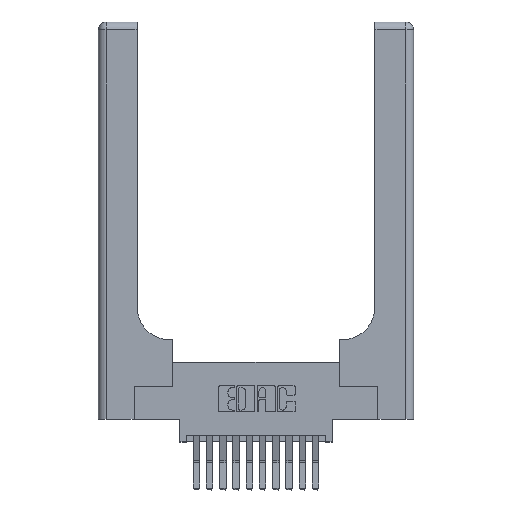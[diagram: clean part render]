
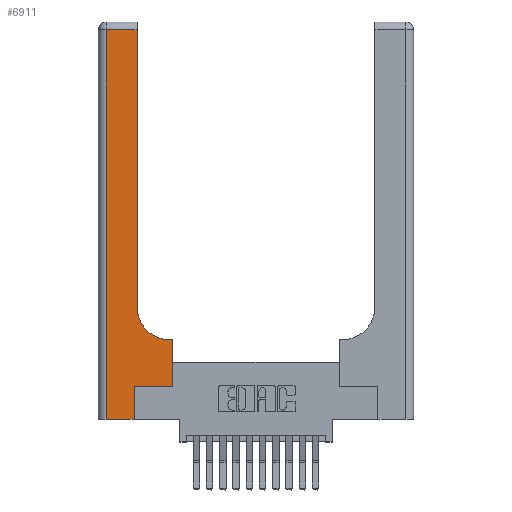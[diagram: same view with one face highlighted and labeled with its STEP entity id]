
A CAD part, top view. The second image highlights one B-rep face of the part: STEP entity #6911.
In plain terms, the highlighted planar face has unit normal (0, 0, 1).
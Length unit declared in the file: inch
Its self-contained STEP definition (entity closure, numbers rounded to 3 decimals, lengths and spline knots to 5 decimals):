
#152 = ORIENTED_EDGE ( 'NONE', *, *, #15202, .T. ) ;
#239 = ORIENTED_EDGE ( 'NONE', *, *, #14470, .T. ) ;
#265 = ORIENTED_EDGE ( 'NONE', *, *, #12878, .T. ) ;
#397 = ORIENTED_EDGE ( 'NONE', *, *, #15425, .T. ) ;
#580 = CARTESIAN_POINT ( 'NONE',  ( 0.269, 0., 0.37 ) ) ;
#607 = CARTESIAN_POINT ( 'NONE',  ( 0.2915, 3., 0.37 ) ) ;
#729 = ORIENTED_EDGE ( 'NONE', *, *, #12782, .T. ) ;
#766 = VECTOR ( 'NONE', #2302, 39.37008 ) ;
#855 = ORIENTED_EDGE ( 'NONE', *, *, #3325, .T. ) ;
#947 = ORIENTED_EDGE ( 'NONE', *, *, #1879, .T. ) ;
#1004 = ORIENTED_EDGE ( 'NONE', *, *, #9409, .T. ) ;
#1080 = ORIENTED_EDGE ( 'NONE', *, *, #13594, .T. ) ;
#1739 = CARTESIAN_POINT ( 'NONE',  ( 0.5585, 0.25, 0.37 ) ) ;
#1879 = EDGE_CURVE ( 'NONE', #11825, #15811, #7840, .T. ) ;
#2097 = VECTOR ( 'NONE', #4702, 39.37008 ) ;
#2302 = DIRECTION ( 'NONE',  ( 0., -1., 0. ) ) ;
#2559 = VECTOR ( 'NONE', #10254, 39.37008 ) ;
#2686 = VECTOR ( 'NONE', #6074, 39.37008 ) ;
#2848 = CARTESIAN_POINT ( 'NONE',  ( 0.06, 2.94, 0.37 ) ) ;
#3325 = EDGE_CURVE ( 'NONE', #12259, #11825, #9900, .T. ) ;
#3659 = CARTESIAN_POINT ( 'NONE',  ( 0.269, 0.25, 0.37 ) ) ;
#3710 = DIRECTION ( 'NONE',  ( 1., 0., 0. ) ) ;
#3801 = CARTESIAN_POINT ( 'NONE',  ( 0., 0., 0.37 ) ) ;
#3952 = CARTESIAN_POINT ( 'NONE',  ( 0.5415, 0.6, 0.37 ) ) ;
#4039 = DIRECTION ( 'NONE',  ( 0., 0., -1. ) ) ;
#4230 = VERTEX_POINT ( 'NONE', #2848 ) ;
#4231 = VERTEX_POINT ( 'NONE', #14883 ) ;
#4249 = VECTOR ( 'NONE', #15240, 39.37008 ) ;
#4646 = LINE ( 'NONE', #607, #15344 ) ;
#4690 = VERTEX_POINT ( 'NONE', #3952 ) ;
#4702 = DIRECTION ( 'NONE',  ( -1., 0., 0. ) ) ;
#4704 = CARTESIAN_POINT ( 'NONE',  ( 0.2915, 0.6, 0.37 ) ) ;
#5261 = LINE ( 'NONE', #3801, #8450 ) ;
#5728 = LINE ( 'NONE', #8730, #2097 ) ;
#6055 = EDGE_LOOP ( 'NONE', ( #152, #239, #265, #397, #729, #855, #947, #1004, #1080 ) ) ;
#6074 = DIRECTION ( 'NONE',  ( -1., 0., 0. ) ) ;
#6312 = VECTOR ( 'NONE', #3710, 39.37008 ) ;
#6911 = ADVANCED_FACE ( 'NONE', ( #14519 ), #11009, .F. ) ;
#7008 = DIRECTION ( 'NONE',  ( 0., 0., -1. ) ) ;
#7840 = LINE ( 'NONE', #1739, #4249 ) ;
#7886 = AXIS2_PLACEMENT_3D ( 'NONE', #12119, #4039, #13439 ) ;
#8450 = VECTOR ( 'NONE', #15857, 39.37008 ) ;
#8522 = CIRCLE ( 'NONE', #7886, 0.25 ) ;
#8603 = CARTESIAN_POINT ( 'NONE',  ( 0.06, 0., 0.37 ) ) ;
#8730 = CARTESIAN_POINT ( 'NONE',  ( 0., 2.94, 0.37 ) ) ;
#8832 = CARTESIAN_POINT ( 'NONE',  ( 0.2915, 2.94, 0.37 ) ) ;
#9090 = CARTESIAN_POINT ( 'NONE',  ( 0.5585, 0.25, 0.37 ) ) ;
#9343 = LINE ( 'NONE', #10425, #766 ) ;
#9409 = EDGE_CURVE ( 'NONE', #15811, #4690, #13433, .T. ) ;
#9900 = LINE ( 'NONE', #3659, #6312 ) ;
#10172 = DIRECTION ( 'NONE',  ( 0., 1., 0. ) ) ;
#10254 = DIRECTION ( 'NONE',  ( 0., 1., 0. ) ) ;
#10425 = CARTESIAN_POINT ( 'NONE',  ( 0.06, 3., 0.37 ) ) ;
#11009 = PLANE ( 'NONE',  #14548 ) ;
#11076 = VERTEX_POINT ( 'NONE', #8832 ) ;
#11682 = CARTESIAN_POINT ( 'NONE',  ( 0.269, 0.25, 0.37 ) ) ;
#11825 = VERTEX_POINT ( 'NONE', #9090 ) ;
#12119 = CARTESIAN_POINT ( 'NONE',  ( 0.5415, 0.85, 0.37 ) ) ;
#12259 = VERTEX_POINT ( 'NONE', #11682 ) ;
#12357 = CARTESIAN_POINT ( 'NONE',  ( 0., 3., 0.37 ) ) ;
#12588 = VERTEX_POINT ( 'NONE', #8603 ) ;
#12782 = EDGE_CURVE ( 'NONE', #16269, #12259, #16428, .T. ) ;
#12878 = EDGE_CURVE ( 'NONE', #4230, #12588, #9343, .T. ) ;
#12962 = CARTESIAN_POINT ( 'NONE',  ( 0.269, 0., 0.37 ) ) ;
#13433 = LINE ( 'NONE', #4704, #2686 ) ;
#13439 = DIRECTION ( 'NONE',  ( 1., 0., 0. ) ) ;
#13594 = EDGE_CURVE ( 'NONE', #4690, #4231, #8522, .T. ) ;
#14470 = EDGE_CURVE ( 'NONE', #11076, #4230, #5728, .T. ) ;
#14519 = FACE_OUTER_BOUND ( 'NONE', #6055, .T. ) ;
#14548 = AXIS2_PLACEMENT_3D ( 'NONE', #12357, #7008, #16340 ) ;
#14883 = CARTESIAN_POINT ( 'NONE',  ( 0.2915, 0.85, 0.37 ) ) ;
#15202 = EDGE_CURVE ( 'NONE', #4231, #11076, #4646, .T. ) ;
#15240 = DIRECTION ( 'NONE',  ( 0., 1., 0. ) ) ;
#15344 = VECTOR ( 'NONE', #10172, 39.37008 ) ;
#15425 = EDGE_CURVE ( 'NONE', #12588, #16269, #5261, .T. ) ;
#15791 = CARTESIAN_POINT ( 'NONE',  ( 0.5585, 0.6, 0.37 ) ) ;
#15811 = VERTEX_POINT ( 'NONE', #15791 ) ;
#15857 = DIRECTION ( 'NONE',  ( 1., 0., 0. ) ) ;
#16269 = VERTEX_POINT ( 'NONE', #580 ) ;
#16340 = DIRECTION ( 'NONE',  ( -1., 0., 0. ) ) ;
#16428 = LINE ( 'NONE', #12962, #2559 ) ;
